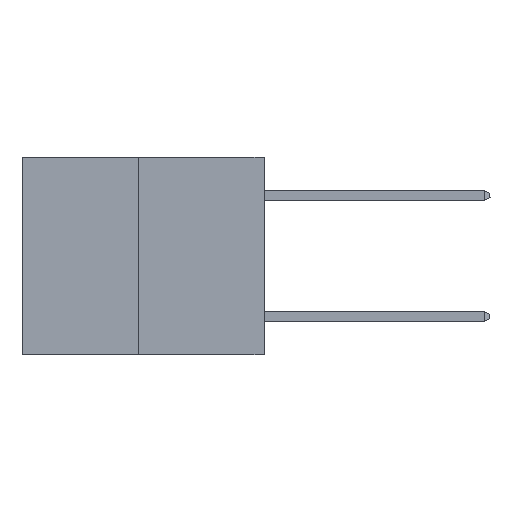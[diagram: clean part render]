
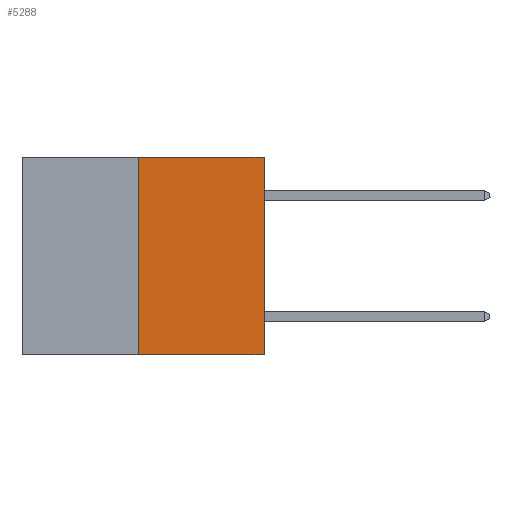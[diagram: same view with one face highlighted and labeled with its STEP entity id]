
A CAD part, left-side view. The second image highlights one B-rep face of the part: STEP entity #5288.
In plain terms, the highlighted planar face has unit normal (-1, 0, 0).
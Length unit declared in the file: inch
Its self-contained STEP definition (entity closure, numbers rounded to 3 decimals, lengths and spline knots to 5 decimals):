
#1140 = VERTEX_POINT ( 'NONE', #7322 ) ;
#2909 = ORIENTED_EDGE ( 'NONE', *, *, #18177, .F. ) ;
#4627 = VERTEX_POINT ( 'NONE', #12817 ) ;
#5288 = ADVANCED_FACE ( 'NONE', ( #7257 ), #20042, .F. ) ;
#5370 = CARTESIAN_POINT ( 'NONE',  ( 0., 0.312, 0. ) ) ;
#5616 = VERTEX_POINT ( 'NONE', #12133 ) ;
#5806 = CARTESIAN_POINT ( 'NONE',  ( 0., 0.6, -0.49 ) ) ;
#6442 = CARTESIAN_POINT ( 'NONE',  ( 0., 0.312, -0.49 ) ) ;
#7257 = FACE_OUTER_BOUND ( 'NONE', #12727, .T. ) ;
#7322 = CARTESIAN_POINT ( 'NONE',  ( 0., 0., 0. ) ) ;
#8061 = CARTESIAN_POINT ( 'NONE',  ( 0., 0.6, 0. ) ) ;
#8336 = VECTOR ( 'NONE', #12436, 39.37008 ) ;
#11779 = ORIENTED_EDGE ( 'NONE', *, *, #12055, .T. ) ;
#12055 = EDGE_CURVE ( 'NONE', #4627, #5616, #15039, .T. ) ;
#12133 = CARTESIAN_POINT ( 'NONE',  ( 0., 0., -0.49 ) ) ;
#12219 = DIRECTION ( 'NONE',  ( 0., -1., 0. ) ) ;
#12436 = DIRECTION ( 'NONE',  ( 0., 0., 1. ) ) ;
#12727 = EDGE_LOOP ( 'NONE', ( #20458, #11779, #23587, #2909 ) ) ;
#12817 = CARTESIAN_POINT ( 'NONE',  ( 0., 0.312, -0.49 ) ) ;
#13104 = EDGE_CURVE ( 'NONE', #4627, #21585, #20464, .T. ) ;
#13848 = DIRECTION ( 'NONE',  ( 0., -1., 0. ) ) ;
#14028 = VECTOR ( 'NONE', #20251, 39.37008 ) ;
#14122 = DIRECTION ( 'NONE',  ( 1., 0., 0. ) ) ;
#15039 = LINE ( 'NONE', #5806, #22116 ) ;
#15995 = DIRECTION ( 'NONE',  ( 0., 0., -1. ) ) ;
#16322 = AXIS2_PLACEMENT_3D ( 'NONE', #8061, #14122, #15995 ) ;
#17192 = LINE ( 'NONE', #24459, #8336 ) ;
#18177 = EDGE_CURVE ( 'NONE', #21585, #1140, #24191, .T. ) ;
#20042 = PLANE ( 'NONE',  #16322 ) ;
#20251 = DIRECTION ( 'NONE',  ( 0., 0., 1. ) ) ;
#20458 = ORIENTED_EDGE ( 'NONE', *, *, #13104, .F. ) ;
#20464 = LINE ( 'NONE', #6442, #14028 ) ;
#21585 = VERTEX_POINT ( 'NONE', #5370 ) ;
#22116 = VECTOR ( 'NONE', #13848, 39.37008 ) ;
#22634 = VECTOR ( 'NONE', #12219, 39.37008 ) ;
#23587 = ORIENTED_EDGE ( 'NONE', *, *, #25292, .T. ) ;
#24191 = LINE ( 'NONE', #24426, #22634 ) ;
#24426 = CARTESIAN_POINT ( 'NONE',  ( 0., 0.6, 0. ) ) ;
#24459 = CARTESIAN_POINT ( 'NONE',  ( 0., 0., 0. ) ) ;
#25292 = EDGE_CURVE ( 'NONE', #5616, #1140, #17192, .T. ) ;
